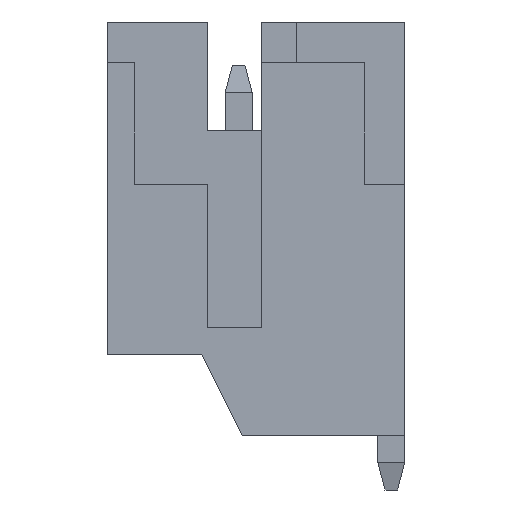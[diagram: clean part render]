
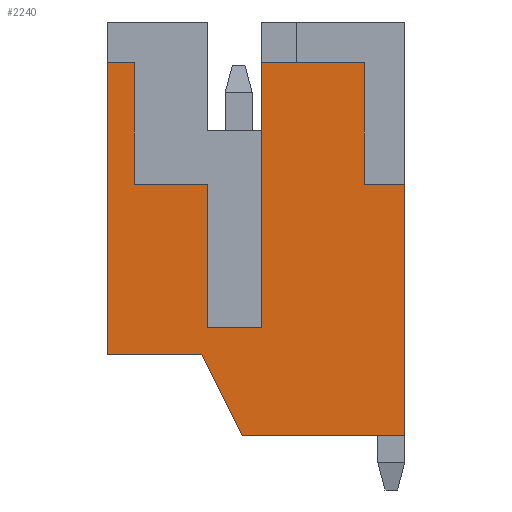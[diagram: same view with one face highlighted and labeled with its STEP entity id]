
A CAD part, left-side view. The second image highlights one B-rep face of the part: STEP entity #2240.
In plain terms, the highlighted planar face has unit normal (-1, 0, 0).
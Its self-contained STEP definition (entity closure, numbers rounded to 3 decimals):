
#23 = ORIENTED_EDGE ( 'NONE', *, *, #3159, .T. ) ;
#62 = VERTEX_POINT ( 'NONE', #1399 ) ;
#66 = DIRECTION ( 'NONE',  ( 0., 0., 1. ) ) ;
#131 = LINE ( 'NONE', #5642, #2116 ) ;
#441 = DIRECTION ( 'NONE',  ( 0., 0., 1. ) ) ;
#466 = CARTESIAN_POINT ( 'NONE',  ( -3., 1.93, 5.4 ) ) ;
#580 = DIRECTION ( 'NONE',  ( 0., -1., 0. ) ) ;
#629 = EDGE_CURVE ( 'NONE', #7456, #2822, #5625, .T. ) ;
#708 = ORIENTED_EDGE ( 'NONE', *, *, #1802, .T. ) ;
#763 = CARTESIAN_POINT ( 'NONE',  ( -3., -3.07, 5.4 ) ) ;
#782 = CARTESIAN_POINT ( 'NONE',  ( -3., 2.43, 6.15 ) ) ;
#816 = LINE ( 'NONE', #4984, #4704 ) ;
#900 = EDGE_CURVE ( 'NONE', #7713, #7440, #816, .T. ) ;
#932 = ORIENTED_EDGE ( 'NONE', *, *, #2425, .T. ) ;
#1022 = CARTESIAN_POINT ( 'NONE',  ( -3., 0.58, 3.15 ) ) ;
#1102 = CARTESIAN_POINT ( 'NONE',  ( -3., 0.68, 0. ) ) ;
#1116 = EDGE_CURVE ( 'NONE', #7216, #7109, #6997, .T. ) ;
#1185 = CARTESIAN_POINT ( 'NONE',  ( -3., 0.58, 3.15 ) ) ;
#1188 = DIRECTION ( 'NONE',  ( -1., 0., 0. ) ) ;
#1271 = EDGE_LOOP ( 'NONE', ( #3203, #932, #7298, #1668, #2685, #5571, #1454, #23, #1685, #7641, #5368, #4204, #4063, #708 ) ) ;
#1399 = CARTESIAN_POINT ( 'NONE',  ( -3., 1.93, 3.15 ) ) ;
#1454 = ORIENTED_EDGE ( 'NONE', *, *, #5524, .F. ) ;
#1525 = EDGE_CURVE ( 'NONE', #7440, #5381, #4907, .T. ) ;
#1574 = CARTESIAN_POINT ( 'NONE',  ( -3., -0.42, 3.15 ) ) ;
#1668 = ORIENTED_EDGE ( 'NONE', *, *, #4651, .T. ) ;
#1685 = ORIENTED_EDGE ( 'NONE', *, *, #2826, .T. ) ;
#1802 = EDGE_CURVE ( 'NONE', #62, #7456, #4255, .T. ) ;
#1908 = CARTESIAN_POINT ( 'NONE',  ( -3., -2.32, 5.4 ) ) ;
#2025 = CARTESIAN_POINT ( 'NONE',  ( -3., -0.42, 0.5 ) ) ;
#2040 = VECTOR ( 'NONE', #8076, 1000. ) ;
#2094 = CARTESIAN_POINT ( 'NONE',  ( -3., 2.43, 0. ) ) ;
#2116 = VECTOR ( 'NONE', #4256, 1000. ) ;
#2183 = VERTEX_POINT ( 'NONE', #1102 ) ;
#2240 = ADVANCED_FACE ( 'NONE', ( #8435 ), #7321, .T. ) ;
#2253 = VECTOR ( 'NONE', #441, 1000. ) ;
#2336 = CARTESIAN_POINT ( 'NONE',  ( -3., -3.07, -1.5 ) ) ;
#2392 = LINE ( 'NONE', #2736, #8368 ) ;
#2425 = EDGE_CURVE ( 'NONE', #2822, #2929, #4571, .T. ) ;
#2663 = LINE ( 'NONE', #2667, #6439 ) ;
#2667 = CARTESIAN_POINT ( 'NONE',  ( -3., -3.07, 5.4 ) ) ;
#2685 = ORIENTED_EDGE ( 'NONE', *, *, #900, .T. ) ;
#2736 = CARTESIAN_POINT ( 'NONE',  ( -3., -2.32, 3.15 ) ) ;
#2822 = VERTEX_POINT ( 'NONE', #8055 ) ;
#2826 = EDGE_CURVE ( 'NONE', #6501, #7216, #2663, .T. ) ;
#2845 = CARTESIAN_POINT ( 'NONE',  ( -3., -0.42, 5.4 ) ) ;
#2929 = VERTEX_POINT ( 'NONE', #4491 ) ;
#3011 = VECTOR ( 'NONE', #3868, 1000. ) ;
#3159 = EDGE_CURVE ( 'NONE', #6001, #6501, #6645, .T. ) ;
#3203 = ORIENTED_EDGE ( 'NONE', *, *, #629, .T. ) ;
#3353 = DIRECTION ( 'NONE',  ( 0., 1., 0. ) ) ;
#3610 = VECTOR ( 'NONE', #4645, 1000. ) ;
#3639 = DIRECTION ( 'NONE',  ( 0., -1., 0. ) ) ;
#3796 = EDGE_CURVE ( 'NONE', #6482, #7109, #131, .T. ) ;
#3868 = DIRECTION ( 'NONE',  ( 0., 0., -1. ) ) ;
#4063 = ORIENTED_EDGE ( 'NONE', *, *, #8658, .F. ) ;
#4204 = ORIENTED_EDGE ( 'NONE', *, *, #5404, .F. ) ;
#4246 = VECTOR ( 'NONE', #6177, 1000. ) ;
#4255 = LINE ( 'NONE', #8464, #2253 ) ;
#4256 = DIRECTION ( 'NONE',  ( 0., -1., 0. ) ) ;
#4491 = CARTESIAN_POINT ( 'NONE',  ( -3., 2.43, 0. ) ) ;
#4528 = CARTESIAN_POINT ( 'NONE',  ( -3., -0.07, -1.5 ) ) ;
#4571 = LINE ( 'NONE', #782, #4246 ) ;
#4645 = DIRECTION ( 'NONE',  ( 0., 0., 1. ) ) ;
#4651 = EDGE_CURVE ( 'NONE', #2183, #7713, #8592, .T. ) ;
#4704 = VECTOR ( 'NONE', #3639, 1000. ) ;
#4779 = DIRECTION ( 'NONE',  ( 0., -1., 0. ) ) ;
#4892 = DIRECTION ( 'NONE',  ( 0., -1., 0. ) ) ;
#4907 = LINE ( 'NONE', #6635, #5851 ) ;
#4984 = CARTESIAN_POINT ( 'NONE',  ( -3., -3.07, -1.5 ) ) ;
#5338 = CARTESIAN_POINT ( 'NONE',  ( -3., -2.32, 3.15 ) ) ;
#5368 = ORIENTED_EDGE ( 'NONE', *, *, #3796, .F. ) ;
#5381 = VERTEX_POINT ( 'NONE', #7147 ) ;
#5404 = EDGE_CURVE ( 'NONE', #7560, #6482, #5984, .T. ) ;
#5524 = EDGE_CURVE ( 'NONE', #6001, #5381, #2392, .T. ) ;
#5571 = ORIENTED_EDGE ( 'NONE', *, *, #1525, .T. ) ;
#5625 = LINE ( 'NONE', #763, #2040 ) ;
#5642 = CARTESIAN_POINT ( 'NONE',  ( -3., -0.42, 0.5 ) ) ;
#5759 = AXIS2_PLACEMENT_3D ( 'NONE', #7837, #1188, #580 ) ;
#5832 = VECTOR ( 'NONE', #4892, 1000. ) ;
#5851 = VECTOR ( 'NONE', #66, 1000. ) ;
#5885 = VECTOR ( 'NONE', #7171, 1000. ) ;
#5963 = CARTESIAN_POINT ( 'NONE',  ( -3., -2.32, 3.15 ) ) ;
#5984 = LINE ( 'NONE', #1185, #5885 ) ;
#6001 = VERTEX_POINT ( 'NONE', #5338 ) ;
#6146 = EDGE_CURVE ( 'NONE', #2929, #2183, #8567, .T. ) ;
#6177 = DIRECTION ( 'NONE',  ( 0., 0., -1. ) ) ;
#6357 = CARTESIAN_POINT ( 'NONE',  ( -3., -0.07, -1.5 ) ) ;
#6439 = VECTOR ( 'NONE', #3353, 1000. ) ;
#6482 = VERTEX_POINT ( 'NONE', #6652 ) ;
#6501 = VERTEX_POINT ( 'NONE', #1908 ) ;
#6526 = CARTESIAN_POINT ( 'NONE',  ( -3., -0.42, 6.15 ) ) ;
#6635 = CARTESIAN_POINT ( 'NONE',  ( -3., -3.07, 6.15 ) ) ;
#6645 = LINE ( 'NONE', #5963, #3610 ) ;
#6652 = CARTESIAN_POINT ( 'NONE',  ( -3., 0.58, 0.5 ) ) ;
#6758 = LINE ( 'NONE', #1574, #5832 ) ;
#6787 = VECTOR ( 'NONE', #4779, 1000. ) ;
#6823 = VECTOR ( 'NONE', #7789, 1000. ) ;
#6997 = LINE ( 'NONE', #6526, #3011 ) ;
#7109 = VERTEX_POINT ( 'NONE', #2025 ) ;
#7147 = CARTESIAN_POINT ( 'NONE',  ( -3., -3.07, 3.15 ) ) ;
#7171 = DIRECTION ( 'NONE',  ( 0., 0., -1. ) ) ;
#7216 = VERTEX_POINT ( 'NONE', #2845 ) ;
#7298 = ORIENTED_EDGE ( 'NONE', *, *, #6146, .T. ) ;
#7321 = PLANE ( 'NONE',  #5759 ) ;
#7440 = VERTEX_POINT ( 'NONE', #2336 ) ;
#7456 = VERTEX_POINT ( 'NONE', #466 ) ;
#7560 = VERTEX_POINT ( 'NONE', #1022 ) ;
#7641 = ORIENTED_EDGE ( 'NONE', *, *, #1116, .T. ) ;
#7713 = VERTEX_POINT ( 'NONE', #4528 ) ;
#7789 = DIRECTION ( 'NONE',  ( 0., -0.447, -0.894 ) ) ;
#7837 = CARTESIAN_POINT ( 'NONE',  ( -3., 0., 0. ) ) ;
#8055 = CARTESIAN_POINT ( 'NONE',  ( -3., 2.43, 5.4 ) ) ;
#8076 = DIRECTION ( 'NONE',  ( 0., 1., 0. ) ) ;
#8093 = DIRECTION ( 'NONE',  ( 0., -1., 0. ) ) ;
#8368 = VECTOR ( 'NONE', #8093, 1000. ) ;
#8435 = FACE_OUTER_BOUND ( 'NONE', #1271, .T. ) ;
#8464 = CARTESIAN_POINT ( 'NONE',  ( -3., 1.93, 3.15 ) ) ;
#8567 = LINE ( 'NONE', #2094, #6787 ) ;
#8592 = LINE ( 'NONE', #6357, #6823 ) ;
#8658 = EDGE_CURVE ( 'NONE', #62, #7560, #6758, .T. ) ;
